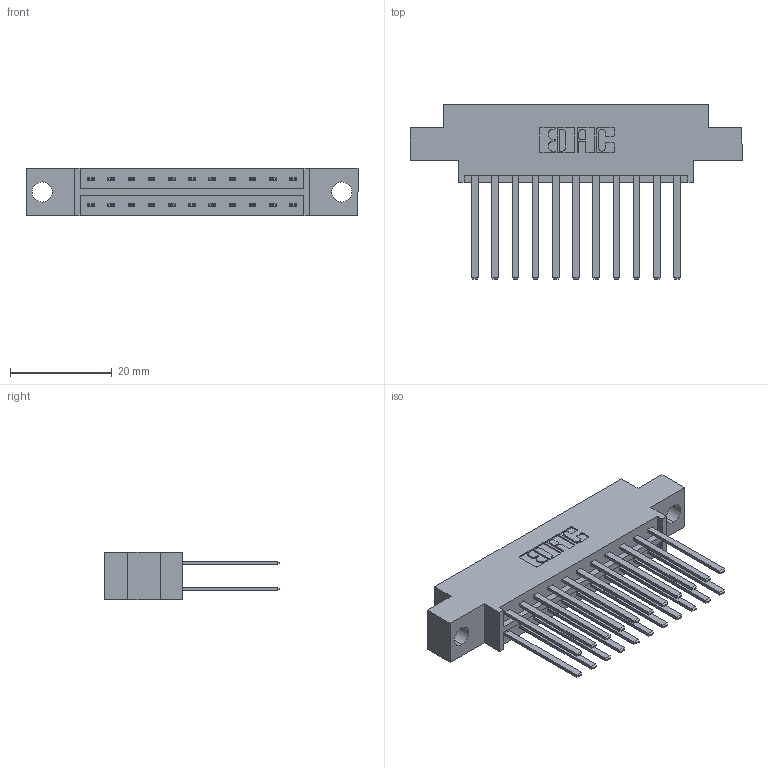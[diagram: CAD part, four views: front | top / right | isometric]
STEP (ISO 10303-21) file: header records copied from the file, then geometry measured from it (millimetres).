
FILE_DESCRIPTION (( 'STEP AP203' ), '1' );
FILE_NAME ('333-022-544-804.STEP', '2018-08-02T02:35:55', ( '' ), ( '' ), 'SwSTEP 2.0', 'SolidWorks 2016', '' );
FILE_SCHEMA (( 'CONFIG_CONTROL_DESIGN' ));
Length unit declared in the file: inch
Products named in the file (3): 333-022-544-804; 333 Part_Offset - .156 Dia - TH; 345-292-001_345-293-144
Assembly tree (23 placements, depth 2):
  333-022-544-804
    333 Part_Offset - .156 Dia - TH
    345-292-001_345-293-144  x22
Bounding box: 65.13 x 34.3 x 9.4 mm (x, y, z)
Volume: 6351.8 mm3; surface area: 8189.5 mm2
Topology: 23 solids, 23 shells, 1130 faces, 3337 edges, 2194 vertices
Faces by surface type: plane 778, cylinder 352
Entity records: 11037 total; most frequent: CARTESIAN_POINT 1866, ORIENTED_EDGE 1802, DIRECTION 1645, EDGE_CURVE 901, LINE 777, VECTOR 777, VERTEX_POINT 598, AXIS2_PLACEMENT_3D 434
